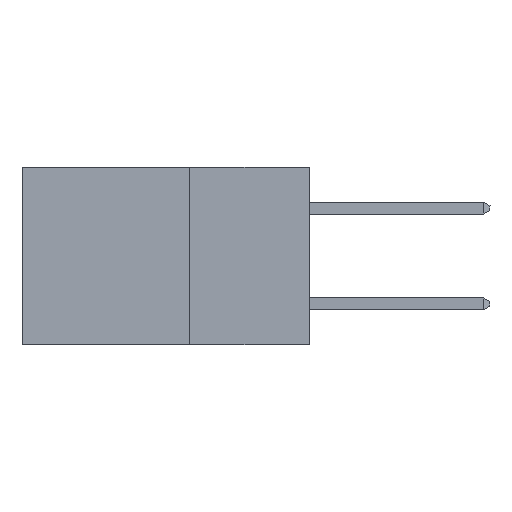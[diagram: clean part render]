
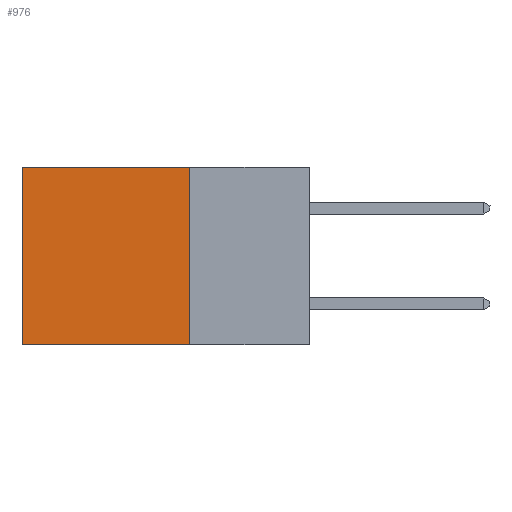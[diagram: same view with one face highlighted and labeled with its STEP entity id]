
A CAD part, left-side view. The second image highlights one B-rep face of the part: STEP entity #976.
In plain terms, the highlighted planar face has unit normal (-1, 0, 0).
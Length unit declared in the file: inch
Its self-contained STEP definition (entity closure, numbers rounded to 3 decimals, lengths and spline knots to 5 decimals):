
#122 = ORIENTED_EDGE ( 'NONE', *, *, #3098, .F. ) ;
#349 = LINE ( 'NONE', #12359, #17947 ) ;
#976 = ADVANCED_FACE ( 'NONE', ( #14344 ), #5177, .F. ) ;
#1973 = CARTESIAN_POINT ( 'NONE',  ( 0.2875, 0.6, 0. ) ) ;
#2540 = ORIENTED_EDGE ( 'NONE', *, *, #8190, .T. ) ;
#2900 = CARTESIAN_POINT ( 'NONE',  ( 0.2875, 0.6, -0.37 ) ) ;
#3051 = LINE ( 'NONE', #13628, #7706 ) ;
#3098 = EDGE_CURVE ( 'NONE', #13460, #12007, #3051, .T. ) ;
#3166 = DIRECTION ( 'NONE',  ( 0., 0., -1. ) ) ;
#4316 = VERTEX_POINT ( 'NONE', #2900 ) ;
#4576 = CARTESIAN_POINT ( 'NONE',  ( 0.2875, 0.25, 0. ) ) ;
#5098 = DIRECTION ( 'NONE',  ( 1., 0., 0. ) ) ;
#5177 = PLANE ( 'NONE',  #22463 ) ;
#5279 = CARTESIAN_POINT ( 'NONE',  ( 0.2875, 0.25, 0. ) ) ;
#6293 = DIRECTION ( 'NONE',  ( 0., 0., -1. ) ) ;
#7515 = EDGE_CURVE ( 'NONE', #12007, #4316, #8488, .T. ) ;
#7706 = VECTOR ( 'NONE', #3166, 39.37008 ) ;
#8190 = EDGE_CURVE ( 'NONE', #13460, #16383, #349, .T. ) ;
#8488 = LINE ( 'NONE', #17540, #17177 ) ;
#9550 = ORIENTED_EDGE ( 'NONE', *, *, #7515, .F. ) ;
#9588 = EDGE_CURVE ( 'NONE', #16383, #4316, #20201, .T. ) ;
#10254 = DIRECTION ( 'NONE',  ( 0., 0., -1. ) ) ;
#11312 = EDGE_LOOP ( 'NONE', ( #15558, #9550, #122, #2540 ) ) ;
#11662 = VECTOR ( 'NONE', #10254, 39.37008 ) ;
#12007 = VERTEX_POINT ( 'NONE', #17579 ) ;
#12359 = CARTESIAN_POINT ( 'NONE',  ( 0.2875, 0.25, 0. ) ) ;
#13460 = VERTEX_POINT ( 'NONE', #4576 ) ;
#13628 = CARTESIAN_POINT ( 'NONE',  ( 0.2875, 0.25, 0. ) ) ;
#14344 = FACE_OUTER_BOUND ( 'NONE', #11312, .T. ) ;
#15558 = ORIENTED_EDGE ( 'NONE', *, *, #9588, .T. ) ;
#16383 = VERTEX_POINT ( 'NONE', #1973 ) ;
#17177 = VECTOR ( 'NONE', #19198, 39.37008 ) ;
#17265 = CARTESIAN_POINT ( 'NONE',  ( 0.2875, 0.6, 0. ) ) ;
#17540 = CARTESIAN_POINT ( 'NONE',  ( 0.2875, 0.25, -0.37 ) ) ;
#17579 = CARTESIAN_POINT ( 'NONE',  ( 0.2875, 0.25, -0.37 ) ) ;
#17947 = VECTOR ( 'NONE', #19171, 39.37008 ) ;
#19171 = DIRECTION ( 'NONE',  ( 0., 1., 0. ) ) ;
#19198 = DIRECTION ( 'NONE',  ( 0., 1., 0. ) ) ;
#20201 = LINE ( 'NONE', #17265, #11662 ) ;
#22463 = AXIS2_PLACEMENT_3D ( 'NONE', #5279, #5098, #6293 ) ;
